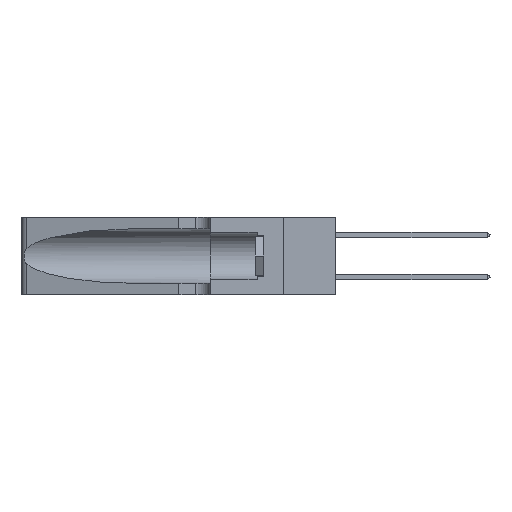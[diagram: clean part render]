
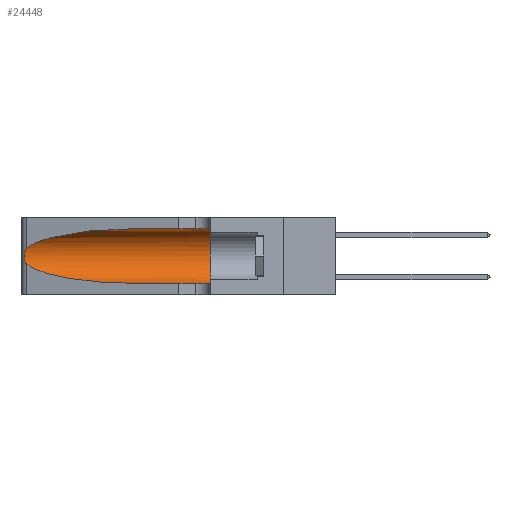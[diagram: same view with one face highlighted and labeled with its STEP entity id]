
A CAD part, left-side view. The second image highlights one B-rep face of the part: STEP entity #24448.
In plain terms, the highlighted cylindrical face has radius 3.308 mm (diameter 6.617 mm), a partial arc.
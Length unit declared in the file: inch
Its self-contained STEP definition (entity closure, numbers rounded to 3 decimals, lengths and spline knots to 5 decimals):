
#25 = VECTOR ( 'NONE', #1721, 39.37008 ) ;
#36 = CARTESIAN_POINT ( 'NONE',  ( 0.18966, 0.96281, 0.05475 ) ) ;
#394 = CARTESIAN_POINT ( 'NONE',  ( 0.25789, 1.23486, 0.15765 ) ) ;
#807 = DIRECTION ( 'NONE',  ( 0., 1., 0. ) ) ;
#1440 = VERTEX_POINT ( 'NONE', #32485 ) ;
#1721 = DIRECTION ( 'NONE',  ( 0., -1., 0. ) ) ;
#3416 = CARTESIAN_POINT ( 'NONE',  ( 0.25555, 1.22993, 0.14849 ) ) ;
#3700 = CARTESIAN_POINT ( 'NONE',  ( 0.25487, 1.22718, 0.22369 ) ) ;
#3770 = EDGE_CURVE ( 'NONE', #31737, #1440, #4441, .T. ) ;
#4108 = CARTESIAN_POINT ( 'NONE',  ( 0.1305, 1.61858, 0.185 ) ) ;
#4441 = B_SPLINE_CURVE_WITH_KNOTS ( 'NONE', 3,
 ( #20526, #28915, #26184, #9212, #29042, #12137, #31884, #14974, #34697, #17802, #394, #20651, #3416, #23466 ),
 .UNSPECIFIED., .F., .F.,
 ( 4, 2, 2, 2, 2, 2, 4 ),
 ( 0., 0.00027, 0.00053, 0.00107, 0.0016, 0.00187, 0.00214 ),
 .UNSPECIFIED. ) ;
#5955 = ORIENTED_EDGE ( 'NONE', *, *, #20731, .F. ) ;
#7227 = EDGE_CURVE ( 'NONE', #15809, #31737, #15137, .T. ) ;
#7331 = EDGE_CURVE ( 'NONE', #1440, #28211, #8472, .T. ) ;
#7714 = CYLINDRICAL_SURFACE ( 'NONE', #25534, 0.13025 ) ;
#8263 = CARTESIAN_POINT ( 'NONE',  ( 0.18966, 0.96281, 0.31525 ) ) ;
#8385 = CARTESIAN_POINT ( 'NONE',  ( 0.2373, 1.15595, 0.28018 ) ) ;
#8472 =( BOUNDED_CURVE ( )  B_SPLINE_CURVE ( 3, ( #34382, #14668, #36, #20331 ),
 .UNSPECIFIED., .F., .F. ) 
 B_SPLINE_CURVE_WITH_KNOTS ( ( 4, 4 ),
 ( 3.44316, 4.71239 ),
 .UNSPECIFIED. ) 
 CURVE ( )  GEOMETRIC_REPRESENTATION_ITEM ( )  RATIONAL_B_SPLINE_CURVE ( ( 1., 0.87, 0.87, 1. ) ) 
 REPRESENTATION_ITEM ( '' )  );
#8849 = ORIENTED_EDGE ( 'NONE', *, *, #7331, .T. ) ;
#9212 = CARTESIAN_POINT ( 'NONE',  ( 0.25787, 1.23484, 0.2124 ) ) ;
#9723 = CARTESIAN_POINT ( 'NONE',  ( 0.1305, 0.35, 0.05475 ) ) ;
#12137 = CARTESIAN_POINT ( 'NONE',  ( 0.26018, 1.23835, 0.19895 ) ) ;
#13830 = ORIENTED_EDGE ( 'NONE', *, *, #3770, .T. ) ;
#14047 = CARTESIAN_POINT ( 'NONE',  ( 0.1305, 0.72297, 0.31525 ) ) ;
#14668 = CARTESIAN_POINT ( 'NONE',  ( 0.2373, 1.15595, 0.08982 ) ) ;
#14719 = LINE ( 'NONE', #35958, #25 ) ;
#14974 = CARTESIAN_POINT ( 'NONE',  ( 0.26075, 1.23896, 0.178 ) ) ;
#15137 =( BOUNDED_CURVE ( )  B_SPLINE_CURVE ( 3, ( #14047, #8263, #8385, #28222 ),
 .UNSPECIFIED., .F., .T. ) 
 B_SPLINE_CURVE_WITH_KNOTS ( ( 4, 4 ),
 ( 1.5708, 2.84003 ),
 .UNSPECIFIED. ) 
 CURVE ( )  GEOMETRIC_REPRESENTATION_ITEM ( )  RATIONAL_B_SPLINE_CURVE ( ( 1., 0.87, 0.87, 1. ) ) 
 REPRESENTATION_ITEM ( '' )  );
#15809 = VERTEX_POINT ( 'NONE', #20141 ) ;
#17296 = EDGE_CURVE ( 'NONE', #18791, #26293, #27350, .T. ) ;
#17802 = CARTESIAN_POINT ( 'NONE',  ( 0.25856, 1.23593, 0.16098 ) ) ;
#18064 = EDGE_CURVE ( 'NONE', #28211, #26293, #29968, .T. ) ;
#18176 = CARTESIAN_POINT ( 'NONE',  ( 0.1305, 0.35, 0.185 ) ) ;
#18459 = DIRECTION ( 'NONE',  ( 0., 0., -1. ) ) ;
#18747 = CARTESIAN_POINT ( 'NONE',  ( 0.1305, 1.61858, 0.05475 ) ) ;
#18791 = VERTEX_POINT ( 'NONE', #22404 ) ;
#18797 = AXIS2_PLACEMENT_3D ( 'NONE', #18176, #807, #21034 ) ;
#20141 = CARTESIAN_POINT ( 'NONE',  ( 0.1305, 0.72297, 0.31525 ) ) ;
#20331 = CARTESIAN_POINT ( 'NONE',  ( 0.1305, 0.72297, 0.05475 ) ) ;
#20526 = CARTESIAN_POINT ( 'NONE',  ( 0.25487, 1.22718, 0.22369 ) ) ;
#20651 = CARTESIAN_POINT ( 'NONE',  ( 0.25639, 1.23186, 0.15144 ) ) ;
#20731 = EDGE_CURVE ( 'NONE', #15809, #18791, #14719, .T. ) ;
#21034 = DIRECTION ( 'NONE',  ( 0., 0., 1. ) ) ;
#21576 = VECTOR ( 'NONE', #32941, 39.37008 ) ;
#22263 = ORIENTED_EDGE ( 'NONE', *, *, #17296, .F. ) ;
#22404 = CARTESIAN_POINT ( 'NONE',  ( 0.1305, 0.35, 0.31525 ) ) ;
#23466 = CARTESIAN_POINT ( 'NONE',  ( 0.25487, 1.22718, 0.14631 ) ) ;
#24012 = DIRECTION ( 'NONE',  ( 0., -1., 0. ) ) ;
#24192 = EDGE_LOOP ( 'NONE', ( #24237, #13830, #8849, #35955, #22263, #5955 ) ) ;
#24237 = ORIENTED_EDGE ( 'NONE', *, *, #7227, .T. ) ;
#24448 = ADVANCED_FACE ( 'NONE', ( #31255 ), #7714, .F. ) ;
#25534 = AXIS2_PLACEMENT_3D ( 'NONE', #4108, #24012, #18459 ) ;
#26184 = CARTESIAN_POINT ( 'NONE',  ( 0.25639, 1.23184, 0.21858 ) ) ;
#26293 = VERTEX_POINT ( 'NONE', #9723 ) ;
#27350 = CIRCLE ( 'NONE', #18797, 0.13025 ) ;
#28211 = VERTEX_POINT ( 'NONE', #35498 ) ;
#28222 = CARTESIAN_POINT ( 'NONE',  ( 0.25487, 1.22718, 0.22369 ) ) ;
#28915 = CARTESIAN_POINT ( 'NONE',  ( 0.25555, 1.22994, 0.2215 ) ) ;
#29042 = CARTESIAN_POINT ( 'NONE',  ( 0.25854, 1.2359, 0.20912 ) ) ;
#29968 = LINE ( 'NONE', #18747, #21576 ) ;
#31255 = FACE_OUTER_BOUND ( 'NONE', #24192, .T. ) ;
#31737 = VERTEX_POINT ( 'NONE', #3700 ) ;
#31884 = CARTESIAN_POINT ( 'NONE',  ( 0.26075, 1.23896, 0.19203 ) ) ;
#32485 = CARTESIAN_POINT ( 'NONE',  ( 0.25487, 1.22718, 0.14631 ) ) ;
#32941 = DIRECTION ( 'NONE',  ( 0., -1., 0. ) ) ;
#34382 = CARTESIAN_POINT ( 'NONE',  ( 0.25487, 1.22718, 0.14631 ) ) ;
#34697 = CARTESIAN_POINT ( 'NONE',  ( 0.26017, 1.23833, 0.17102 ) ) ;
#35498 = CARTESIAN_POINT ( 'NONE',  ( 0.1305, 0.72297, 0.05475 ) ) ;
#35955 = ORIENTED_EDGE ( 'NONE', *, *, #18064, .T. ) ;
#35958 = CARTESIAN_POINT ( 'NONE',  ( 0.1305, 1.61858, 0.31525 ) ) ;
